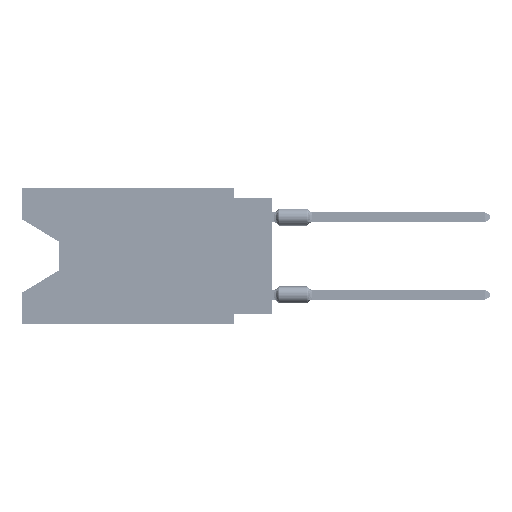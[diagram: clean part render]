
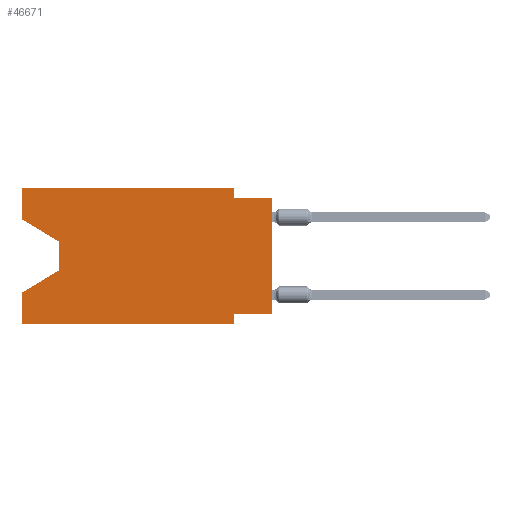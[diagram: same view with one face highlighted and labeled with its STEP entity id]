
A CAD part, left-side view. The second image highlights one B-rep face of the part: STEP entity #46671.
In plain terms, the highlighted planar face has unit normal (-1, 0, 0).
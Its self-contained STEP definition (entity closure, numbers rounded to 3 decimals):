
#646 = CARTESIAN_POINT ( 'NONE',  ( 0., 16.383, -8.89 ) ) ;
#899 = ORIENTED_EDGE ( 'NONE', *, *, #22099, .T. ) ;
#1043 = CARTESIAN_POINT ( 'NONE',  ( 0., 16.383, 0. ) ) ;
#1329 = CARTESIAN_POINT ( 'NONE',  ( 0., 16.383, 0. ) ) ;
#1779 = VERTEX_POINT ( 'NONE', #19667 ) ;
#2470 = ORIENTED_EDGE ( 'NONE', *, *, #61962, .F. ) ;
#2512 = VECTOR ( 'NONE', #37933, 1000. ) ;
#3091 = DIRECTION ( 'NONE',  ( 0., 0., 1. ) ) ;
#5045 = VECTOR ( 'NONE', #74607, 1000. ) ;
#8571 = EDGE_CURVE ( 'NONE', #86968, #13545, #44504, .T. ) ;
#9511 = VERTEX_POINT ( 'NONE', #70268 ) ;
#9964 = CARTESIAN_POINT ( 'NONE',  ( 0., 16.383, 0. ) ) ;
#11036 = CARTESIAN_POINT ( 'NONE',  ( 0., 0., 0. ) ) ;
#11085 = EDGE_CURVE ( 'NONE', #86968, #23293, #64173, .T. ) ;
#11368 = DIRECTION ( 'NONE',  ( 0., 0., -1. ) ) ;
#13463 = ORIENTED_EDGE ( 'NONE', *, *, #65021, .F. ) ;
#13545 = VERTEX_POINT ( 'NONE', #84025 ) ;
#13960 = LINE ( 'NONE', #89151, #61252 ) ;
#14761 = LINE ( 'NONE', #43303, #61317 ) ;
#14906 = ORIENTED_EDGE ( 'NONE', *, *, #28641, .F. ) ;
#16719 = ORIENTED_EDGE ( 'NONE', *, *, #79310, .F. ) ;
#17188 = DIRECTION ( 'NONE',  ( 0., 0., -1. ) ) ;
#17278 = VERTEX_POINT ( 'NONE', #40637 ) ;
#18018 = VECTOR ( 'NONE', #3091, 1000. ) ;
#18044 = LINE ( 'NONE', #11036, #18018 ) ;
#19417 = VECTOR ( 'NONE', #36131, 1000. ) ;
#19667 = CARTESIAN_POINT ( 'NONE',  ( 0., 2.54, -0.635 ) ) ;
#22099 = EDGE_CURVE ( 'NONE', #67059, #17278, #18044, .T. ) ;
#22649 = DIRECTION ( 'NONE',  ( 0., -1., 0. ) ) ;
#23293 = VERTEX_POINT ( 'NONE', #88299 ) ;
#24497 = CARTESIAN_POINT ( 'NONE',  ( 0., 2.54, -8.89 ) ) ;
#24918 = DIRECTION ( 'NONE',  ( 1., 0., 0. ) ) ;
#25807 = CARTESIAN_POINT ( 'NONE',  ( 0., 16.383, -8.89 ) ) ;
#26381 = CARTESIAN_POINT ( 'NONE',  ( 0., 0., -8.255 ) ) ;
#26493 = VECTOR ( 'NONE', #43142, 1000. ) ;
#27741 = VECTOR ( 'NONE', #22649, 1000. ) ;
#27913 = CARTESIAN_POINT ( 'NONE',  ( 0., 2.54, -8.89 ) ) ;
#28046 = DIRECTION ( 'NONE',  ( 0., -1., 0. ) ) ;
#28641 = EDGE_CURVE ( 'NONE', #63534, #64687, #46457, .T. ) ;
#29672 = CARTESIAN_POINT ( 'NONE',  ( 0., 16.383, -2.038 ) ) ;
#30388 = AXIS2_PLACEMENT_3D ( 'NONE', #9964, #24918, #74448 ) ;
#31116 = LINE ( 'NONE', #68023, #73144 ) ;
#35498 = ORIENTED_EDGE ( 'NONE', *, *, #48797, .T. ) ;
#35669 = CARTESIAN_POINT ( 'NONE',  ( 0., 16.383, 0. ) ) ;
#36131 = DIRECTION ( 'NONE',  ( 0., -1., 0. ) ) ;
#36409 = LINE ( 'NONE', #38087, #81335 ) ;
#37933 = DIRECTION ( 'NONE',  ( 0., -0.855, -0.519 ) ) ;
#38087 = CARTESIAN_POINT ( 'NONE',  ( 0., 0., -0.635 ) ) ;
#38593 = DIRECTION ( 'NONE',  ( 0., 1., 0. ) ) ;
#39859 = FACE_OUTER_BOUND ( 'NONE', #47305, .T. ) ;
#40637 = CARTESIAN_POINT ( 'NONE',  ( 0., 0., -0.635 ) ) ;
#43142 = DIRECTION ( 'NONE',  ( 0., 0., 1. ) ) ;
#43303 = CARTESIAN_POINT ( 'NONE',  ( 0., 13.97, -5.385 ) ) ;
#43893 = LINE ( 'NONE', #1329, #55034 ) ;
#44128 = LINE ( 'NONE', #646, #27741 ) ;
#44504 = LINE ( 'NONE', #58970, #2512 ) ;
#45191 = ORIENTED_EDGE ( 'NONE', *, *, #47946, .F. ) ;
#45743 = ORIENTED_EDGE ( 'NONE', *, *, #8571, .T. ) ;
#46457 = LINE ( 'NONE', #24497, #69913 ) ;
#46480 = EDGE_CURVE ( 'NONE', #13545, #82609, #52199, .T. ) ;
#46671 = ADVANCED_FACE ( 'NONE', ( #39859 ), #88467, .F. ) ;
#47305 = EDGE_LOOP ( 'NONE', ( #45743, #87506, #70156, #2470, #35498, #14906, #13463, #899, #45191, #82162, #16719, #49633 ) ) ;
#47946 = EDGE_CURVE ( 'NONE', #1779, #17278, #36409, .T. ) ;
#48797 = EDGE_CURVE ( 'NONE', #88864, #64687, #44128, .T. ) ;
#49633 = ORIENTED_EDGE ( 'NONE', *, *, #11085, .F. ) ;
#50615 = LINE ( 'NONE', #1043, #19417 ) ;
#52199 = LINE ( 'NONE', #59667, #5045 ) ;
#55034 = VECTOR ( 'NONE', #87790, 1000. ) ;
#57502 = CARTESIAN_POINT ( 'NONE',  ( 0., 13.97, -5.385 ) ) ;
#58114 = CARTESIAN_POINT ( 'NONE',  ( 0., 2.54, -8.255 ) ) ;
#58970 = CARTESIAN_POINT ( 'NONE',  ( 0., 16.383, -2.038 ) ) ;
#59667 = CARTESIAN_POINT ( 'NONE',  ( 0., 13.97, -3.505 ) ) ;
#61252 = VECTOR ( 'NONE', #17188, 1000. ) ;
#61317 = VECTOR ( 'NONE', #64781, 1000. ) ;
#61962 = EDGE_CURVE ( 'NONE', #88864, #9511, #43893, .T. ) ;
#63534 = VERTEX_POINT ( 'NONE', #58114 ) ;
#64173 = LINE ( 'NONE', #35669, #26493 ) ;
#64687 = VERTEX_POINT ( 'NONE', #27913 ) ;
#64781 = DIRECTION ( 'NONE',  ( 0., 0.855, -0.519 ) ) ;
#65021 = EDGE_CURVE ( 'NONE', #67059, #63534, #31116, .T. ) ;
#67059 = VERTEX_POINT ( 'NONE', #26381 ) ;
#68023 = CARTESIAN_POINT ( 'NONE',  ( 0., 0., -8.255 ) ) ;
#69913 = VECTOR ( 'NONE', #11368, 1000. ) ;
#70156 = ORIENTED_EDGE ( 'NONE', *, *, #81902, .T. ) ;
#70268 = CARTESIAN_POINT ( 'NONE',  ( 0., 16.383, -6.852 ) ) ;
#73144 = VECTOR ( 'NONE', #38593, 1000. ) ;
#74448 = DIRECTION ( 'NONE',  ( 0., 0., -1. ) ) ;
#74607 = DIRECTION ( 'NONE',  ( 0., 0., -1. ) ) ;
#79310 = EDGE_CURVE ( 'NONE', #23293, #88201, #50615, .T. ) ;
#80124 = CARTESIAN_POINT ( 'NONE',  ( 0., 2.54, 0. ) ) ;
#81335 = VECTOR ( 'NONE', #28046, 1000. ) ;
#81486 = EDGE_CURVE ( 'NONE', #88201, #1779, #13960, .T. ) ;
#81902 = EDGE_CURVE ( 'NONE', #82609, #9511, #14761, .T. ) ;
#82162 = ORIENTED_EDGE ( 'NONE', *, *, #81486, .F. ) ;
#82609 = VERTEX_POINT ( 'NONE', #57502 ) ;
#84025 = CARTESIAN_POINT ( 'NONE',  ( 0., 13.97, -3.505 ) ) ;
#86968 = VERTEX_POINT ( 'NONE', #29672 ) ;
#87506 = ORIENTED_EDGE ( 'NONE', *, *, #46480, .T. ) ;
#87790 = DIRECTION ( 'NONE',  ( 0., 0., 1. ) ) ;
#88201 = VERTEX_POINT ( 'NONE', #80124 ) ;
#88299 = CARTESIAN_POINT ( 'NONE',  ( 0., 16.383, 0. ) ) ;
#88467 = PLANE ( 'NONE',  #30388 ) ;
#88864 = VERTEX_POINT ( 'NONE', #25807 ) ;
#89151 = CARTESIAN_POINT ( 'NONE',  ( 0., 2.54, 0. ) ) ;
